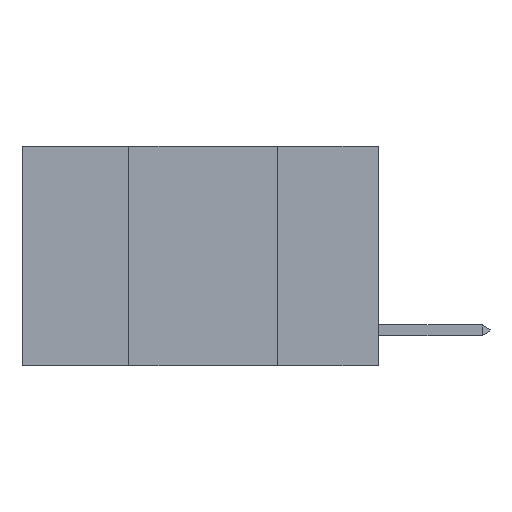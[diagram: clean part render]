
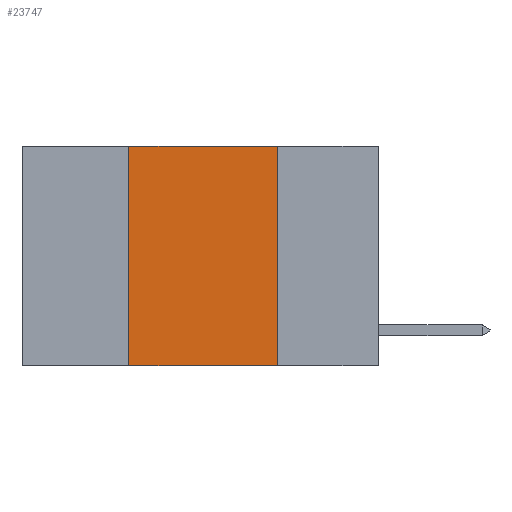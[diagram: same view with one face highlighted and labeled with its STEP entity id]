
A CAD part, left-side view. The second image highlights one B-rep face of the part: STEP entity #23747.
In plain terms, the highlighted planar face has unit normal (-1, 0, 0).
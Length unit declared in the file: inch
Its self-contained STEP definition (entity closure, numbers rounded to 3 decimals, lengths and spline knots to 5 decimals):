
#399 = DIRECTION ( 'NONE',  ( 0., 0., 1. ) ) ;
#866 = ORIENTED_EDGE ( 'NONE', *, *, #6892, .F. ) ;
#1376 = VECTOR ( 'NONE', #1983, 39.37008 ) ;
#1983 = DIRECTION ( 'NONE',  ( 0., -1., 0. ) ) ;
#3177 = CARTESIAN_POINT ( 'NONE',  ( 0., 0.42, 0. ) ) ;
#3492 = CARTESIAN_POINT ( 'NONE',  ( 0., 0.17, 0. ) ) ;
#3578 = DIRECTION ( 'NONE',  ( 1., 0., 0. ) ) ;
#3690 = DIRECTION ( 'NONE',  ( 0., -1., 0. ) ) ;
#3796 = ORIENTED_EDGE ( 'NONE', *, *, #26136, .F. ) ;
#4145 = EDGE_CURVE ( 'NONE', #7555, #14559, #21103, .T. ) ;
#4475 = EDGE_LOOP ( 'NONE', ( #10800, #866, #3796, #11274 ) ) ;
#6138 = LINE ( 'NONE', #17387, #1376 ) ;
#6892 = EDGE_CURVE ( 'NONE', #17262, #7555, #21586, .T. ) ;
#7555 = VERTEX_POINT ( 'NONE', #9694 ) ;
#9694 = CARTESIAN_POINT ( 'NONE',  ( 0., 0.17, 0. ) ) ;
#10800 = ORIENTED_EDGE ( 'NONE', *, *, #4145, .F. ) ;
#11274 = ORIENTED_EDGE ( 'NONE', *, *, #20817, .T. ) ;
#14559 = VERTEX_POINT ( 'NONE', #29034 ) ;
#14680 = CARTESIAN_POINT ( 'NONE',  ( 0., 0.6, 0. ) ) ;
#14933 = AXIS2_PLACEMENT_3D ( 'NONE', #14680, #3578, #21189 ) ;
#16002 = VECTOR ( 'NONE', #399, 39.37008 ) ;
#16511 = LINE ( 'NONE', #3177, #16002 ) ;
#17262 = VERTEX_POINT ( 'NONE', #26344 ) ;
#17387 = CARTESIAN_POINT ( 'NONE',  ( 0., 0.6, -0.37 ) ) ;
#18165 = CARTESIAN_POINT ( 'NONE',  ( 0., 0.42, -0.37 ) ) ;
#19296 = VECTOR ( 'NONE', #3690, 39.37008 ) ;
#20817 = EDGE_CURVE ( 'NONE', #27326, #14559, #6138, .T. ) ;
#21103 = LINE ( 'NONE', #3492, #25761 ) ;
#21189 = DIRECTION ( 'NONE',  ( 0., 0., -1. ) ) ;
#21586 = LINE ( 'NONE', #23961, #19296 ) ;
#23747 = ADVANCED_FACE ( 'NONE', ( #27675 ), #25764, .F. ) ;
#23961 = CARTESIAN_POINT ( 'NONE',  ( 0., 0.6, 0. ) ) ;
#25541 = DIRECTION ( 'NONE',  ( 0., 0., -1. ) ) ;
#25761 = VECTOR ( 'NONE', #25541, 39.37008 ) ;
#25764 = PLANE ( 'NONE',  #14933 ) ;
#26136 = EDGE_CURVE ( 'NONE', #27326, #17262, #16511, .T. ) ;
#26344 = CARTESIAN_POINT ( 'NONE',  ( 0., 0.42, 0. ) ) ;
#27326 = VERTEX_POINT ( 'NONE', #18165 ) ;
#27675 = FACE_OUTER_BOUND ( 'NONE', #4475, .T. ) ;
#29034 = CARTESIAN_POINT ( 'NONE',  ( 0., 0.17, -0.37 ) ) ;
